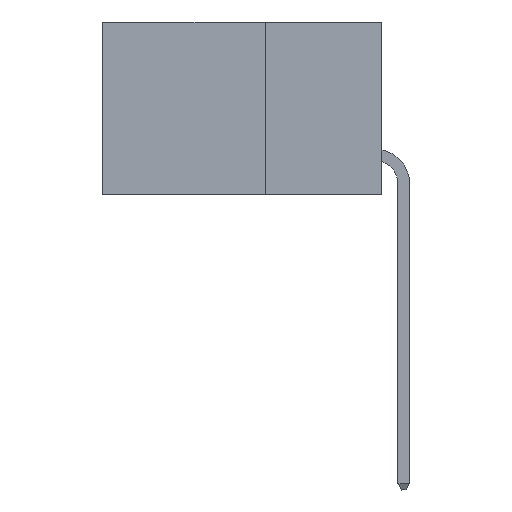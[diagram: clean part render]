
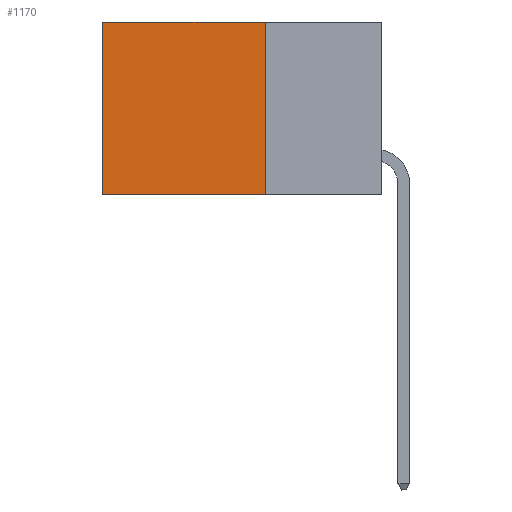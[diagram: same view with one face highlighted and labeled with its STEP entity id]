
A CAD part, left-side view. The second image highlights one B-rep face of the part: STEP entity #1170.
In plain terms, the highlighted planar face has unit normal (-1, 0, 0).
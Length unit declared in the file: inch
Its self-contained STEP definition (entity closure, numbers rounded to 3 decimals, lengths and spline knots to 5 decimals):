
#1097 = DIRECTION ( 'NONE',  ( 0., 1., 0. ) ) ;
#1170 = ADVANCED_FACE ( 'NONE', ( #17373 ), #3178, .F. ) ;
#3178 = PLANE ( 'NONE',  #28878 ) ;
#3496 = DIRECTION ( 'NONE',  ( 0., 0., -1. ) ) ;
#3558 = LINE ( 'NONE', #43249, #22235 ) ;
#3818 = ORIENTED_EDGE ( 'NONE', *, *, #17336, .T. ) ;
#4163 = VERTEX_POINT ( 'NONE', #18473 ) ;
#9519 = VERTEX_POINT ( 'NONE', #32033 ) ;
#10903 = ORIENTED_EDGE ( 'NONE', *, *, #35027, .F. ) ;
#14141 = CARTESIAN_POINT ( 'NONE',  ( 0.2875, 0.25, 0. ) ) ;
#14687 = CARTESIAN_POINT ( 'NONE',  ( 0.2875, 0.6, -0.37 ) ) ;
#15680 = LINE ( 'NONE', #25118, #41912 ) ;
#17336 = EDGE_CURVE ( 'NONE', #4163, #29245, #29996, .T. ) ;
#17373 = FACE_OUTER_BOUND ( 'NONE', #45302, .T. ) ;
#17800 = ORIENTED_EDGE ( 'NONE', *, *, #39544, .T. ) ;
#18473 = CARTESIAN_POINT ( 'NONE',  ( 0.2875, 0.6, 0. ) ) ;
#21393 = CARTESIAN_POINT ( 'NONE',  ( 0.2875, 0.6, 0. ) ) ;
#22235 = VECTOR ( 'NONE', #45753, 39.37008 ) ;
#23523 = VECTOR ( 'NONE', #32321, 39.37008 ) ;
#24611 = CARTESIAN_POINT ( 'NONE',  ( 0.2875, 0.25, 0. ) ) ;
#24814 = DIRECTION ( 'NONE',  ( 0., 0., -1. ) ) ;
#25118 = CARTESIAN_POINT ( 'NONE',  ( 0.2875, 0.25, 0. ) ) ;
#27267 = VERTEX_POINT ( 'NONE', #14141 ) ;
#28878 = AXIS2_PLACEMENT_3D ( 'NONE', #40540, #32551, #3496 ) ;
#29035 = ORIENTED_EDGE ( 'NONE', *, *, #43754, .F. ) ;
#29245 = VERTEX_POINT ( 'NONE', #14687 ) ;
#29996 = LINE ( 'NONE', #21393, #36415 ) ;
#32033 = CARTESIAN_POINT ( 'NONE',  ( 0.2875, 0.25, -0.37 ) ) ;
#32321 = DIRECTION ( 'NONE',  ( 0., 0., -1. ) ) ;
#32551 = DIRECTION ( 'NONE',  ( 1., 0., 0. ) ) ;
#33608 = LINE ( 'NONE', #24611, #23523 ) ;
#35027 = EDGE_CURVE ( 'NONE', #27267, #9519, #33608, .T. ) ;
#36415 = VECTOR ( 'NONE', #24814, 39.37008 ) ;
#39544 = EDGE_CURVE ( 'NONE', #27267, #4163, #15680, .T. ) ;
#40540 = CARTESIAN_POINT ( 'NONE',  ( 0.2875, 0.25, 0. ) ) ;
#41912 = VECTOR ( 'NONE', #1097, 39.37008 ) ;
#43249 = CARTESIAN_POINT ( 'NONE',  ( 0.2875, 0.25, -0.37 ) ) ;
#43754 = EDGE_CURVE ( 'NONE', #9519, #29245, #3558, .T. ) ;
#45302 = EDGE_LOOP ( 'NONE', ( #3818, #29035, #10903, #17800 ) ) ;
#45753 = DIRECTION ( 'NONE',  ( 0., 1., 0. ) ) ;
